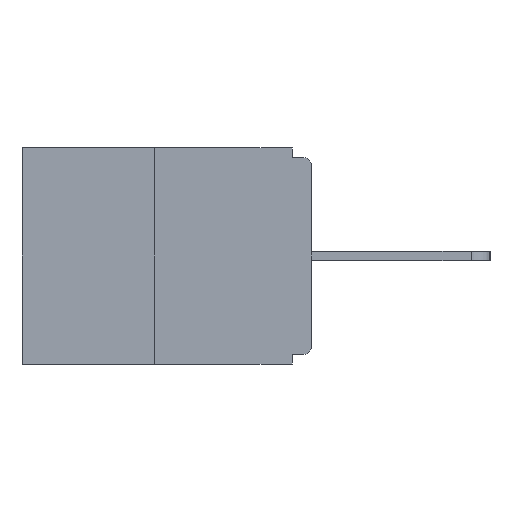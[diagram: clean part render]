
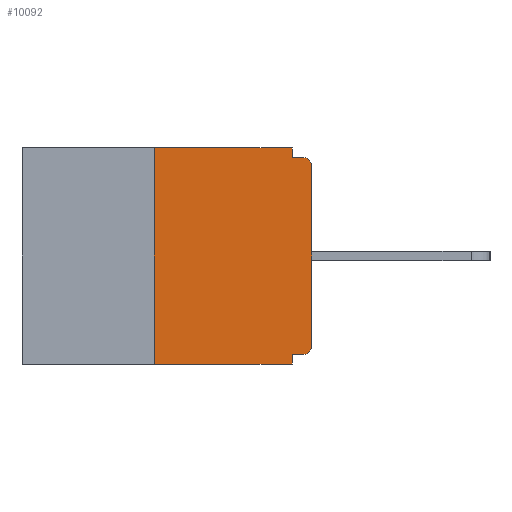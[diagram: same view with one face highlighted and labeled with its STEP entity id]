
A CAD part, left-side view. The second image highlights one B-rep face of the part: STEP entity #10092.
In plain terms, the highlighted planar face has unit normal (-1, 0, 0).
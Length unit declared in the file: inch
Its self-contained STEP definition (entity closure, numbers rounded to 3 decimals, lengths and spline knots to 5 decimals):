
#272 = EDGE_CURVE ( 'NONE', #2900, #21208, #22395, .T. ) ;
#822 = VERTEX_POINT ( 'NONE', #16488 ) ;
#1064 = LINE ( 'NONE', #8052, #1938 ) ;
#1066 = EDGE_CURVE ( 'NONE', #8530, #822, #1064, .T. ) ;
#1127 = ORIENTED_EDGE ( 'NONE', *, *, #13072, .T. ) ;
#1135 = CARTESIAN_POINT ( 'NONE',  ( 0., 0.031, -0.343 ) ) ;
#1459 = ORIENTED_EDGE ( 'NONE', *, *, #1066, .F. ) ;
#1938 = VECTOR ( 'NONE', #6326, 39.37008 ) ;
#1957 = CARTESIAN_POINT ( 'NONE',  ( 0., 0., -0.328 ) ) ;
#2052 = LINE ( 'NONE', #10831, #11942 ) ;
#2406 = DIRECTION ( 'NONE',  ( 0., 0., -1. ) ) ;
#2420 = EDGE_CURVE ( 'NONE', #3826, #11487, #13385, .T. ) ;
#2614 = CARTESIAN_POINT ( 'NONE',  ( 0., 0.015, -0.313 ) ) ;
#2900 = VERTEX_POINT ( 'NONE', #18174 ) ;
#3044 = DIRECTION ( 'NONE',  ( 0., -1., 0. ) ) ;
#3049 = AXIS2_PLACEMENT_3D ( 'NONE', #4272, #11327, #7701 ) ;
#3085 = VECTOR ( 'NONE', #5533, 39.37008 ) ;
#3350 = CARTESIAN_POINT ( 'NONE',  ( 0., 0.031, 0. ) ) ;
#3826 = VERTEX_POINT ( 'NONE', #5570 ) ;
#4047 = CARTESIAN_POINT ( 'NONE',  ( 0., 0., 0. ) ) ;
#4272 = CARTESIAN_POINT ( 'NONE',  ( 0., 0.46, 0. ) ) ;
#4710 = VECTOR ( 'NONE', #3044, 39.37008 ) ;
#4853 = CIRCLE ( 'NONE', #17412, 0.015 ) ;
#5533 = DIRECTION ( 'NONE',  ( 0., 0., 1. ) ) ;
#5570 = CARTESIAN_POINT ( 'NONE',  ( 0., 0.25, -0.343 ) ) ;
#5716 = VERTEX_POINT ( 'NONE', #3350 ) ;
#5802 = DIRECTION ( 'NONE',  ( 0., 0., -1. ) ) ;
#5862 = CARTESIAN_POINT ( 'NONE',  ( 0., 0.46, 0. ) ) ;
#5881 = ORIENTED_EDGE ( 'NONE', *, *, #16981, .F. ) ;
#5965 = CIRCLE ( 'NONE', #12647, 0.015 ) ;
#5976 = DIRECTION ( 'NONE',  ( 0., -1., 0. ) ) ;
#6326 = DIRECTION ( 'NONE',  ( 0., -1., 0. ) ) ;
#6668 = ORIENTED_EDGE ( 'NONE', *, *, #8701, .F. ) ;
#6917 = LINE ( 'NONE', #1957, #10916 ) ;
#7701 = DIRECTION ( 'NONE',  ( 0., 0., -1. ) ) ;
#8052 = CARTESIAN_POINT ( 'NONE',  ( 0., 0., -0.015 ) ) ;
#8530 = VERTEX_POINT ( 'NONE', #16667 ) ;
#8701 = EDGE_CURVE ( 'NONE', #20302, #2900, #6917, .T. ) ;
#8903 = CARTESIAN_POINT ( 'NONE',  ( 0., 0.25, 0. ) ) ;
#8928 = EDGE_CURVE ( 'NONE', #11487, #5716, #21951, .T. ) ;
#9293 = VECTOR ( 'NONE', #14682, 39.37008 ) ;
#9688 = LINE ( 'NONE', #4047, #9293 ) ;
#9963 = LINE ( 'NONE', #22466, #4710 ) ;
#10092 = ADVANCED_FACE ( 'NONE', ( #14913 ), #21623, .F. ) ;
#10704 = CARTESIAN_POINT ( 'NONE',  ( 0., 0., -0.03 ) ) ;
#10831 = CARTESIAN_POINT ( 'NONE',  ( 0., 0.031, 0. ) ) ;
#10916 = VECTOR ( 'NONE', #17464, 39.37008 ) ;
#11162 = EDGE_CURVE ( 'NONE', #20302, #21726, #4853, .T. ) ;
#11327 = DIRECTION ( 'NONE',  ( 1., 0., 0. ) ) ;
#11333 = CARTESIAN_POINT ( 'NONE',  ( 0., 0.031, -0.343 ) ) ;
#11487 = VERTEX_POINT ( 'NONE', #8903 ) ;
#11656 = EDGE_CURVE ( 'NONE', #17020, #822, #5965, .T. ) ;
#11942 = VECTOR ( 'NONE', #2406, 39.37008 ) ;
#12647 = AXIS2_PLACEMENT_3D ( 'NONE', #21665, #21769, #5802 ) ;
#13072 = EDGE_CURVE ( 'NONE', #3826, #21208, #9963, .T. ) ;
#13385 = LINE ( 'NONE', #21393, #3085 ) ;
#13728 = VECTOR ( 'NONE', #16425, 39.37008 ) ;
#14417 = CARTESIAN_POINT ( 'NONE',  ( 0., 0.015, -0.328 ) ) ;
#14682 = DIRECTION ( 'NONE',  ( 0., 0., 1. ) ) ;
#14768 = CARTESIAN_POINT ( 'NONE',  ( 0., 0., -0.313 ) ) ;
#14862 = DIRECTION ( 'NONE',  ( -1., 0., 0. ) ) ;
#14913 = FACE_OUTER_BOUND ( 'NONE', #17562, .T. ) ;
#15229 = ORIENTED_EDGE ( 'NONE', *, *, #18370, .T. ) ;
#16381 = ORIENTED_EDGE ( 'NONE', *, *, #11656, .T. ) ;
#16425 = DIRECTION ( 'NONE',  ( 0., 0., -1. ) ) ;
#16488 = CARTESIAN_POINT ( 'NONE',  ( 0., 0.015, -0.015 ) ) ;
#16667 = CARTESIAN_POINT ( 'NONE',  ( 0., 0.031, -0.015 ) ) ;
#16838 = VECTOR ( 'NONE', #5976, 39.37008 ) ;
#16981 = EDGE_CURVE ( 'NONE', #5716, #8530, #2052, .T. ) ;
#17020 = VERTEX_POINT ( 'NONE', #10704 ) ;
#17412 = AXIS2_PLACEMENT_3D ( 'NONE', #2614, #14862, #21796 ) ;
#17464 = DIRECTION ( 'NONE',  ( 0., 1., 0. ) ) ;
#17562 = EDGE_LOOP ( 'NONE', ( #18798, #17631, #1127, #18014, #6668, #18497, #15229, #16381, #1459, #5881 ) ) ;
#17631 = ORIENTED_EDGE ( 'NONE', *, *, #2420, .F. ) ;
#18014 = ORIENTED_EDGE ( 'NONE', *, *, #272, .F. ) ;
#18174 = CARTESIAN_POINT ( 'NONE',  ( 0., 0.031, -0.328 ) ) ;
#18370 = EDGE_CURVE ( 'NONE', #21726, #17020, #9688, .T. ) ;
#18497 = ORIENTED_EDGE ( 'NONE', *, *, #11162, .T. ) ;
#18798 = ORIENTED_EDGE ( 'NONE', *, *, #8928, .F. ) ;
#20302 = VERTEX_POINT ( 'NONE', #14417 ) ;
#21208 = VERTEX_POINT ( 'NONE', #11333 ) ;
#21393 = CARTESIAN_POINT ( 'NONE',  ( 0., 0.25, 0. ) ) ;
#21623 = PLANE ( 'NONE',  #3049 ) ;
#21665 = CARTESIAN_POINT ( 'NONE',  ( 0., 0.015, -0.03 ) ) ;
#21726 = VERTEX_POINT ( 'NONE', #14768 ) ;
#21769 = DIRECTION ( 'NONE',  ( -1., 0., 0. ) ) ;
#21796 = DIRECTION ( 'NONE',  ( 0., 0., -1. ) ) ;
#21951 = LINE ( 'NONE', #5862, #16838 ) ;
#22395 = LINE ( 'NONE', #1135, #13728 ) ;
#22466 = CARTESIAN_POINT ( 'NONE',  ( 0., 0.46, -0.343 ) ) ;
